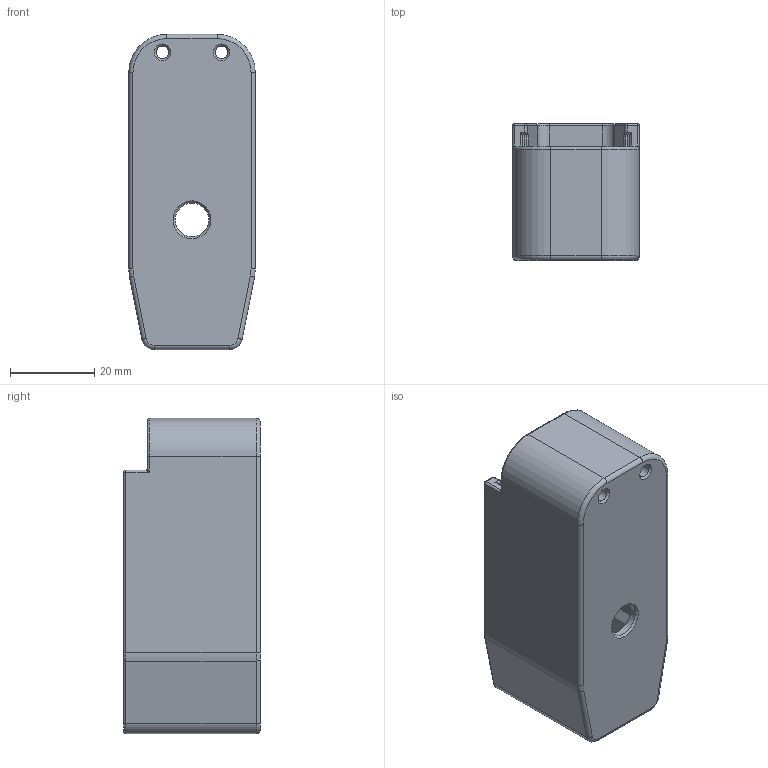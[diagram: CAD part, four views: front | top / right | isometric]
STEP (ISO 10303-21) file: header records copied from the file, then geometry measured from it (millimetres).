
FILE_DESCRIPTION(/* description */ (''),/* implementation_level */ '2;1');
FILE_NAME(/* name */ 'ab437a75-8ae0-41b4-bd3b-0d3e5fde5f36.stp',/* time_stamp */ '2019-04-30T20:32:26-04:00',/* author */ ('suzuki450ltr'),/* organization */ (''),/* preprocessor_version */ 'ST-DEVELOPER v18',/* originating_system */ 'Autodesk Translation Framework v8.2.0.1029',/* authorisation */ '');
FILE_SCHEMA (('AUTOMOTIVE_DESIGN { 1 0 10303 214 3 1 1 }'));
Length unit declared in the file: millimetre
Products named in the file (1): Korean 5.56x45 Mag Extension
Bounding box: 30 x 32.5 x 74.78 mm (x, y, z)
Volume: 33493 mm3; surface area: 15405.8 mm2
Topology: 1 solids, 1 shells, 216 faces, 493 edges, 271 vertices
Faces by surface type: cylinder 106, plane 40, torus 39, bspline 15, sphere 10, cone 6
Full cylindrical faces by diameter (mm): 3 x2, 8 x1
Entity records: 6188 total; most frequent: CARTESIAN_POINT 1237, DIRECTION 1149, ORIENTED_EDGE 968, EDGE_CURVE 484, AXIS2_PLACEMENT_3D 463, VERTEX_POINT 271, CIRCLE 239, LINE 223
